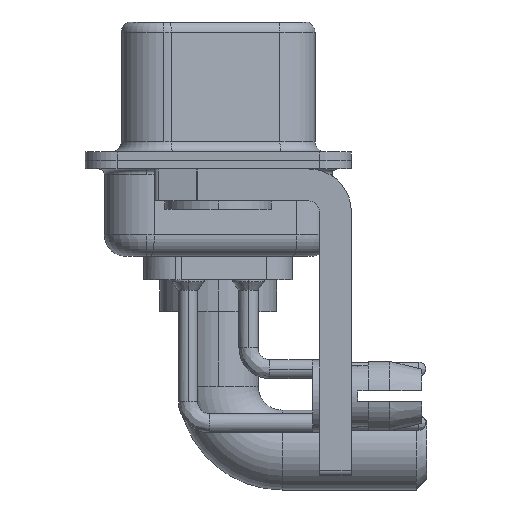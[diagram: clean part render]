
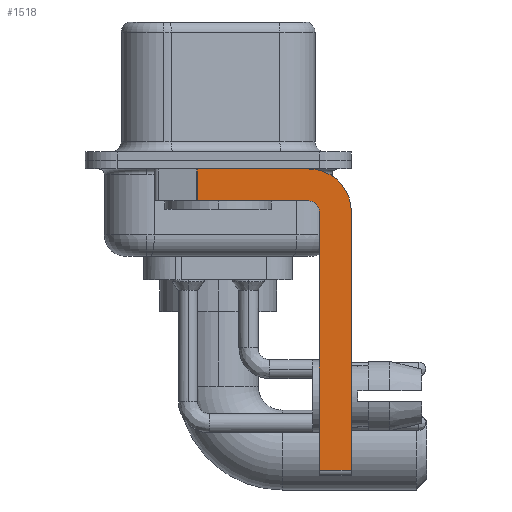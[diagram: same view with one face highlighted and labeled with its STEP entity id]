
A CAD part, left-side view. The second image highlights one B-rep face of the part: STEP entity #1518.
In plain terms, the highlighted planar face has unit normal (-1, 0, 0).
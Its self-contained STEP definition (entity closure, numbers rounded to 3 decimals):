
#157 = VECTOR ( 'NONE', #6694, 1000. ) ;
#1372 = CARTESIAN_POINT ( 'NONE',  ( -2.9, 0.978, -1.9 ) ) ;
#1433 = DIRECTION ( 'NONE',  ( -1., 0., 0. ) ) ;
#1518 = ADVANCED_FACE ( 'NONE', ( #18666 ), #9154, .F. ) ;
#1559 = DIRECTION ( 'NONE',  ( 0., -1., 0. ) ) ;
#1679 = EDGE_CURVE ( 'NONE', #16055, #20526, #13207, .T. ) ;
#2473 = CARTESIAN_POINT ( 'NONE',  ( -2.9, -6.25, -2.4 ) ) ;
#2484 = DIRECTION ( 'NONE',  ( 0., 0., -1. ) ) ;
#2976 = EDGE_CURVE ( 'NONE', #13789, #18401, #3988, .T. ) ;
#3516 = LINE ( 'NONE', #9275, #157 ) ;
#3624 = DIRECTION ( 'NONE',  ( 0., -1., 0. ) ) ;
#3811 = DIRECTION ( 'NONE',  ( 0., 0., 1. ) ) ;
#3988 = LINE ( 'NONE', #17156, #18842 ) ;
#4351 = ORIENTED_EDGE ( 'NONE', *, *, #1679, .F. ) ;
#4542 = ORIENTED_EDGE ( 'NONE', *, *, #21081, .F. ) ;
#4825 = DIRECTION ( 'NONE',  ( 0., 0., 1. ) ) ;
#4827 = EDGE_CURVE ( 'NONE', #20526, #18401, #8120, .T. ) ;
#4991 = CARTESIAN_POINT ( 'NONE',  ( -2.9, 0.978, -0.4 ) ) ;
#5029 = VECTOR ( 'NONE', #1559, 1000. ) ;
#5238 = AXIS2_PLACEMENT_3D ( 'NONE', #9515, #11622, #13498 ) ;
#5294 = ORIENTED_EDGE ( 'NONE', *, *, #6652, .F. ) ;
#5610 = AXIS2_PLACEMENT_3D ( 'NONE', #16787, #7025, #16277 ) ;
#5699 = EDGE_CURVE ( 'NONE', #6791, #10837, #3516, .T. ) ;
#5950 = CARTESIAN_POINT ( 'NONE',  ( -2.9, 3., -0.4 ) ) ;
#6652 = EDGE_CURVE ( 'NONE', #15829, #16055, #11084, .T. ) ;
#6694 = DIRECTION ( 'NONE',  ( 0., 1., 0. ) ) ;
#6766 = CIRCLE ( 'NONE', #14758, 0.5 ) ;
#6791 = VERTEX_POINT ( 'NONE', #21710 ) ;
#7025 = DIRECTION ( 'NONE',  ( 1., 0., 0. ) ) ;
#7126 = ORIENTED_EDGE ( 'NONE', *, *, #5699, .F. ) ;
#8120 = LINE ( 'NONE', #23377, #24535 ) ;
#9154 = PLANE ( 'NONE',  #5610 ) ;
#9193 = EDGE_CURVE ( 'NONE', #15829, #10837, #16406, .T. ) ;
#9275 = CARTESIAN_POINT ( 'NONE',  ( -2.9, -4.25, -1.9 ) ) ;
#9515 = CARTESIAN_POINT ( 'NONE',  ( -2.9, -4.25, -2.4 ) ) ;
#10500 = CARTESIAN_POINT ( 'NONE',  ( -2.9, -6.25, -14.55 ) ) ;
#10837 = VERTEX_POINT ( 'NONE', #12020 ) ;
#11084 = LINE ( 'NONE', #5950, #5029 ) ;
#11415 = EDGE_CURVE ( 'NONE', #11746, #6791, #6766, .T. ) ;
#11622 = DIRECTION ( 'NONE',  ( 1., 0., 0. ) ) ;
#11702 = ORIENTED_EDGE ( 'NONE', *, *, #2976, .T. ) ;
#11746 = VERTEX_POINT ( 'NONE', #20197 ) ;
#12020 = CARTESIAN_POINT ( 'NONE',  ( -2.9, 0.978, -1.9 ) ) ;
#12241 = VECTOR ( 'NONE', #14532, 1000. ) ;
#13114 = CARTESIAN_POINT ( 'NONE',  ( -2.9, -4.25, -0.4 ) ) ;
#13207 = CIRCLE ( 'NONE', #5238, 2. ) ;
#13498 = DIRECTION ( 'NONE',  ( 0., 0., -1. ) ) ;
#13789 = VERTEX_POINT ( 'NONE', #22672 ) ;
#14532 = DIRECTION ( 'NONE',  ( 0., 0., -1. ) ) ;
#14758 = AXIS2_PLACEMENT_3D ( 'NONE', #14840, #1433, #3811 ) ;
#14840 = CARTESIAN_POINT ( 'NONE',  ( -2.9, -4.25, -2.4 ) ) ;
#15287 = ORIENTED_EDGE ( 'NONE', *, *, #9193, .T. ) ;
#15829 = VERTEX_POINT ( 'NONE', #4991 ) ;
#16055 = VERTEX_POINT ( 'NONE', #13114 ) ;
#16277 = DIRECTION ( 'NONE',  ( 0., 0., -1. ) ) ;
#16406 = LINE ( 'NONE', #1372, #12241 ) ;
#16787 = CARTESIAN_POINT ( 'NONE',  ( -2.9, -4.25, -2.4 ) ) ;
#17156 = CARTESIAN_POINT ( 'NONE',  ( -2.9, -4.25, -14.55 ) ) ;
#18401 = VERTEX_POINT ( 'NONE', #10500 ) ;
#18666 = FACE_OUTER_BOUND ( 'NONE', #24722, .T. ) ;
#18842 = VECTOR ( 'NONE', #3624, 1000. ) ;
#18892 = ORIENTED_EDGE ( 'NONE', *, *, #11415, .F. ) ;
#20197 = CARTESIAN_POINT ( 'NONE',  ( -2.9, -4.75, -2.4 ) ) ;
#20526 = VERTEX_POINT ( 'NONE', #2473 ) ;
#21081 = EDGE_CURVE ( 'NONE', #13789, #11746, #21970, .T. ) ;
#21710 = CARTESIAN_POINT ( 'NONE',  ( -2.9, -4.25, -1.9 ) ) ;
#21970 = LINE ( 'NONE', #22090, #22614 ) ;
#22090 = CARTESIAN_POINT ( 'NONE',  ( -2.9, -4.75, -14.8 ) ) ;
#22614 = VECTOR ( 'NONE', #4825, 1000. ) ;
#22672 = CARTESIAN_POINT ( 'NONE',  ( -2.9, -4.75, -14.55 ) ) ;
#23203 = ORIENTED_EDGE ( 'NONE', *, *, #4827, .F. ) ;
#23377 = CARTESIAN_POINT ( 'NONE',  ( -2.9, -6.25, -2.4 ) ) ;
#24535 = VECTOR ( 'NONE', #2484, 1000. ) ;
#24722 = EDGE_LOOP ( 'NONE', ( #5294, #15287, #7126, #18892, #4542, #11702, #23203, #4351 ) ) ;
